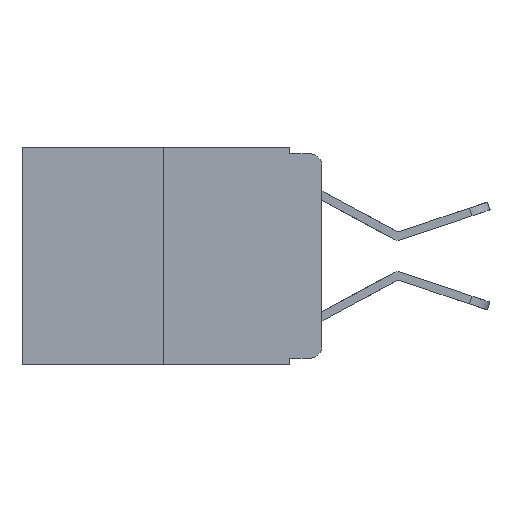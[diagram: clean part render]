
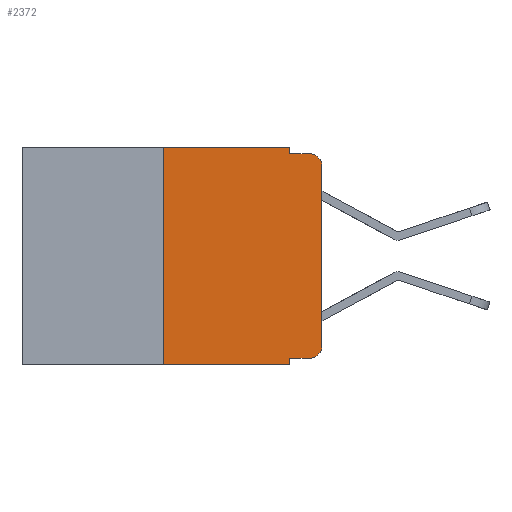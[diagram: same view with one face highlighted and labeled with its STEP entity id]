
A CAD part, left-side view. The second image highlights one B-rep face of the part: STEP entity #2372.
In plain terms, the highlighted planar face has unit normal (-1, 0, 0).
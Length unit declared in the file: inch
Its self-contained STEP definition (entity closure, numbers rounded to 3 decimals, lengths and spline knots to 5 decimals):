
#25 = CARTESIAN_POINT ( 'NONE',  ( 0., 0., 0. ) ) ;
#61 = VECTOR ( 'NONE', #3766, 39.37008 ) ;
#118 = EDGE_CURVE ( 'NONE', #7296, #5318, #8940, .T. ) ;
#373 = DIRECTION ( 'NONE',  ( 0., 0., 1. ) ) ;
#415 = ORIENTED_EDGE ( 'NONE', *, *, #118, .T. ) ;
#536 = VECTOR ( 'NONE', #7359, 39.37008 ) ;
#679 = AXIS2_PLACEMENT_3D ( 'NONE', #7363, #7282, #7210 ) ;
#769 = DIRECTION ( 'NONE',  ( 0., -1., 0. ) ) ;
#857 = ORIENTED_EDGE ( 'NONE', *, *, #11589, .F. ) ;
#975 = FACE_OUTER_BOUND ( 'NONE', #10223, .T. ) ;
#1019 = VERTEX_POINT ( 'NONE', #7673 ) ;
#1163 = EDGE_CURVE ( 'NONE', #1019, #2233, #10956, .T. ) ;
#1177 = ORIENTED_EDGE ( 'NONE', *, *, #11443, .F. ) ;
#1244 = VECTOR ( 'NONE', #373, 39.37008 ) ;
#1265 = AXIS2_PLACEMENT_3D ( 'NONE', #2731, #9336, #3722 ) ;
#1312 = VERTEX_POINT ( 'NONE', #1992 ) ;
#1696 = CARTESIAN_POINT ( 'NONE',  ( 0., 0.051, -0.01 ) ) ;
#1861 = LINE ( 'NONE', #1696, #4197 ) ;
#1992 = CARTESIAN_POINT ( 'NONE',  ( 0., 0.25, 0. ) ) ;
#2233 = VERTEX_POINT ( 'NONE', #7401 ) ;
#2240 = ORIENTED_EDGE ( 'NONE', *, *, #3975, .T. ) ;
#2334 = VERTEX_POINT ( 'NONE', #4547 ) ;
#2372 = ADVANCED_FACE ( 'NONE', ( #975 ), #3797, .F. ) ;
#2454 = CARTESIAN_POINT ( 'NONE',  ( 0., 0.051, -0.343 ) ) ;
#2617 = CARTESIAN_POINT ( 'NONE',  ( 0., 0.051, -0.333 ) ) ;
#2731 = CARTESIAN_POINT ( 'NONE',  ( 0., 0.02, -0.03 ) ) ;
#2771 = CARTESIAN_POINT ( 'NONE',  ( 0., 0.051, 0. ) ) ;
#2853 = CARTESIAN_POINT ( 'NONE',  ( 0., 0.051, -0.333 ) ) ;
#2862 = DIRECTION ( 'NONE',  ( 0., -1., 0. ) ) ;
#2990 = LINE ( 'NONE', #25, #10146 ) ;
#3722 = DIRECTION ( 'NONE',  ( 0., 0., -1. ) ) ;
#3756 = DIRECTION ( 'NONE',  ( 1., 0., 0. ) ) ;
#3766 = DIRECTION ( 'NONE',  ( 0., 0., -1. ) ) ;
#3772 = VERTEX_POINT ( 'NONE', #9635 ) ;
#3797 = PLANE ( 'NONE',  #9117 ) ;
#3975 = EDGE_CURVE ( 'NONE', #5360, #11305, #10569, .T. ) ;
#4047 = CARTESIAN_POINT ( 'NONE',  ( 0., 0.473, 0. ) ) ;
#4197 = VECTOR ( 'NONE', #769, 39.37008 ) ;
#4541 = ORIENTED_EDGE ( 'NONE', *, *, #12023, .F. ) ;
#4547 = CARTESIAN_POINT ( 'NONE',  ( 0., 0., -0.03 ) ) ;
#4626 = LINE ( 'NONE', #6907, #11629 ) ;
#4661 = CIRCLE ( 'NONE', #1265, 0.02 ) ;
#5220 = LINE ( 'NONE', #2771, #61 ) ;
#5318 = VERTEX_POINT ( 'NONE', #8388 ) ;
#5360 = VERTEX_POINT ( 'NONE', #8513 ) ;
#5553 = CARTESIAN_POINT ( 'NONE',  ( 0., 0.051, 0. ) ) ;
#5718 = EDGE_CURVE ( 'NONE', #1312, #1019, #4626, .T. ) ;
#5843 = CARTESIAN_POINT ( 'NONE',  ( 0., 0.473, -0.343 ) ) ;
#5902 = ORIENTED_EDGE ( 'NONE', *, *, #10826, .T. ) ;
#6449 = VECTOR ( 'NONE', #11190, 39.37008 ) ;
#6907 = CARTESIAN_POINT ( 'NONE',  ( 0., 0.473, 0. ) ) ;
#7210 = DIRECTION ( 'NONE',  ( 0., 0., -1. ) ) ;
#7282 = DIRECTION ( 'NONE',  ( -1., 0., 0. ) ) ;
#7296 = VERTEX_POINT ( 'NONE', #9645 ) ;
#7359 = DIRECTION ( 'NONE',  ( 0., -1., 0. ) ) ;
#7363 = CARTESIAN_POINT ( 'NONE',  ( 0., 0.02, -0.313 ) ) ;
#7401 = CARTESIAN_POINT ( 'NONE',  ( 0., 0.051, -0.01 ) ) ;
#7673 = CARTESIAN_POINT ( 'NONE',  ( 0., 0.051, 0. ) ) ;
#7964 = ORIENTED_EDGE ( 'NONE', *, *, #11646, .T. ) ;
#8388 = CARTESIAN_POINT ( 'NONE',  ( 0., 0., -0.313 ) ) ;
#8513 = CARTESIAN_POINT ( 'NONE',  ( 0., 0.25, -0.343 ) ) ;
#8940 = CIRCLE ( 'NONE', #679, 0.02 ) ;
#8988 = CARTESIAN_POINT ( 'NONE',  ( 0., 0.25, 0. ) ) ;
#9117 = AXIS2_PLACEMENT_3D ( 'NONE', #4047, #3756, #11335 ) ;
#9336 = DIRECTION ( 'NONE',  ( -1., 0., 0. ) ) ;
#9573 = DIRECTION ( 'NONE',  ( 0., 0., 1. ) ) ;
#9635 = CARTESIAN_POINT ( 'NONE',  ( 0., 0.02, -0.01 ) ) ;
#9645 = CARTESIAN_POINT ( 'NONE',  ( 0., 0.02, -0.333 ) ) ;
#10146 = VECTOR ( 'NONE', #9573, 39.37008 ) ;
#10223 = EDGE_LOOP ( 'NONE', ( #11144, #5902, #1177, #10590, #11288, #4541, #2240, #857, #7964, #415 ) ) ;
#10246 = EDGE_CURVE ( 'NONE', #5318, #2334, #2990, .T. ) ;
#10381 = LINE ( 'NONE', #8988, #1244 ) ;
#10569 = LINE ( 'NONE', #5843, #536 ) ;
#10590 = ORIENTED_EDGE ( 'NONE', *, *, #1163, .F. ) ;
#10826 = EDGE_CURVE ( 'NONE', #2334, #3772, #4661, .T. ) ;
#10956 = LINE ( 'NONE', #5553, #6449 ) ;
#11144 = ORIENTED_EDGE ( 'NONE', *, *, #10246, .T. ) ;
#11190 = DIRECTION ( 'NONE',  ( 0., 0., -1. ) ) ;
#11211 = DIRECTION ( 'NONE',  ( 0., -1., 0. ) ) ;
#11288 = ORIENTED_EDGE ( 'NONE', *, *, #5718, .F. ) ;
#11305 = VERTEX_POINT ( 'NONE', #2454 ) ;
#11335 = DIRECTION ( 'NONE',  ( 0., 0., -1. ) ) ;
#11366 = VECTOR ( 'NONE', #11211, 39.37008 ) ;
#11385 = VERTEX_POINT ( 'NONE', #2617 ) ;
#11443 = EDGE_CURVE ( 'NONE', #2233, #3772, #1861, .T. ) ;
#11589 = EDGE_CURVE ( 'NONE', #11385, #11305, #5220, .T. ) ;
#11629 = VECTOR ( 'NONE', #2862, 39.37008 ) ;
#11635 = LINE ( 'NONE', #2853, #11366 ) ;
#11646 = EDGE_CURVE ( 'NONE', #11385, #7296, #11635, .T. ) ;
#12023 = EDGE_CURVE ( 'NONE', #5360, #1312, #10381, .T. ) ;
